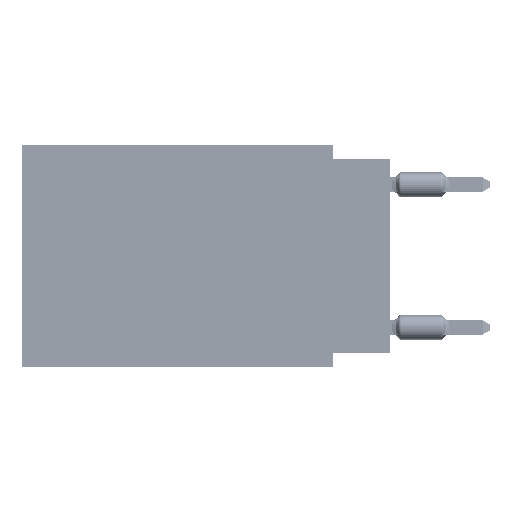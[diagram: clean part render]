
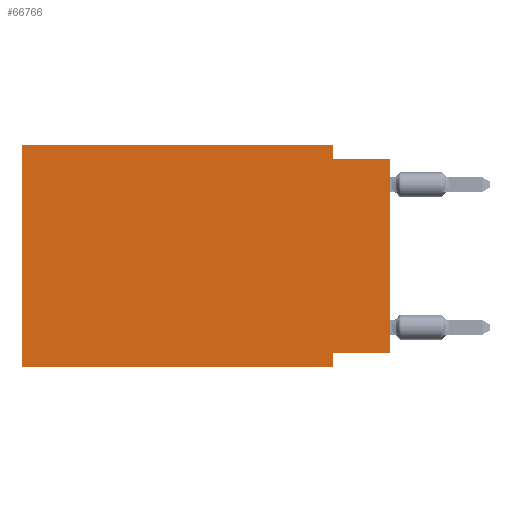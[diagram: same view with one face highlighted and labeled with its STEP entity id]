
A CAD part, left-side view. The second image highlights one B-rep face of the part: STEP entity #66766.
In plain terms, the highlighted planar face has unit normal (-1, 0, 0).
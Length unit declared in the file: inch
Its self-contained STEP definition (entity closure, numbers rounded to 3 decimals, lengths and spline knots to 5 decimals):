
#260 = ORIENTED_EDGE ( 'NONE', *, *, #37451, .T. ) ;
#2139 = DIRECTION ( 'NONE',  ( 0., 0., -1. ) ) ;
#2690 = DIRECTION ( 'NONE',  ( 0., -1., 0. ) ) ;
#2821 = CARTESIAN_POINT ( 'NONE',  ( 0., 0.1, -0.39 ) ) ;
#4115 = VERTEX_POINT ( 'NONE', #2821 ) ;
#4960 = LINE ( 'NONE', #43911, #25141 ) ;
#6924 = ORIENTED_EDGE ( 'NONE', *, *, #10248, .F. ) ;
#7031 = CARTESIAN_POINT ( 'NONE',  ( 0., 0., 0. ) ) ;
#8588 = CARTESIAN_POINT ( 'NONE',  ( 0., 0.1, 0. ) ) ;
#9007 = CARTESIAN_POINT ( 'NONE',  ( 0., 0., -0.025 ) ) ;
#9080 = LINE ( 'NONE', #58769, #21565 ) ;
#9121 = VECTOR ( 'NONE', #60297, 39.37008 ) ;
#9276 = CARTESIAN_POINT ( 'NONE',  ( 0., 0., -0.365 ) ) ;
#9802 = ORIENTED_EDGE ( 'NONE', *, *, #56569, .T. ) ;
#10019 = DIRECTION ( 'NONE',  ( 0., 1., 0. ) ) ;
#10248 = EDGE_CURVE ( 'NONE', #26288, #44771, #20748, .T. ) ;
#11384 = CARTESIAN_POINT ( 'NONE',  ( 0., 0.645, -0.39 ) ) ;
#11724 = CARTESIAN_POINT ( 'NONE',  ( 0., 0.1, 0. ) ) ;
#11728 = CARTESIAN_POINT ( 'NONE',  ( 0., 0.645, -0.39 ) ) ;
#11824 = EDGE_CURVE ( 'NONE', #50966, #15535, #4960, .T. ) ;
#15233 = ORIENTED_EDGE ( 'NONE', *, *, #40867, .F. ) ;
#15535 = VERTEX_POINT ( 'NONE', #11724 ) ;
#15946 = CARTESIAN_POINT ( 'NONE',  ( 0., 0.645, 0. ) ) ;
#15958 = DIRECTION ( 'NONE',  ( 0., 0., 1. ) ) ;
#18775 = CARTESIAN_POINT ( 'NONE',  ( 0., 0., -0.025 ) ) ;
#20002 = EDGE_CURVE ( 'NONE', #15535, #49779, #34676, .T. ) ;
#20748 = LINE ( 'NONE', #42547, #29524 ) ;
#20987 = LINE ( 'NONE', #59203, #32807 ) ;
#21317 = DIRECTION ( 'NONE',  ( 0., 0., -1. ) ) ;
#21565 = VECTOR ( 'NONE', #53057, 39.37008 ) ;
#22765 = LINE ( 'NONE', #7031, #9121 ) ;
#23816 = ORIENTED_EDGE ( 'NONE', *, *, #70513, .F. ) ;
#24324 = VECTOR ( 'NONE', #2139, 39.37008 ) ;
#25141 = VECTOR ( 'NONE', #42475, 39.37008 ) ;
#26288 = VERTEX_POINT ( 'NONE', #9276 ) ;
#28100 = FACE_OUTER_BOUND ( 'NONE', #34383, .T. ) ;
#29524 = VECTOR ( 'NONE', #10019, 39.37008 ) ;
#32807 = VECTOR ( 'NONE', #15958, 39.37008 ) ;
#34383 = EDGE_LOOP ( 'NONE', ( #260, #15233, #36076, #56979, #23816, #9802, #59638, #6924 ) ) ;
#34676 = LINE ( 'NONE', #8588, #24324 ) ;
#36076 = ORIENTED_EDGE ( 'NONE', *, *, #20002, .F. ) ;
#37451 = EDGE_CURVE ( 'NONE', #26288, #57579, #22765, .T. ) ;
#40867 = EDGE_CURVE ( 'NONE', #49779, #57579, #50947, .T. ) ;
#42475 = DIRECTION ( 'NONE',  ( 0., -1., 0. ) ) ;
#42547 = CARTESIAN_POINT ( 'NONE',  ( 0., 0., -0.365 ) ) ;
#43911 = CARTESIAN_POINT ( 'NONE',  ( 0., 0.645, 0. ) ) ;
#44771 = VERTEX_POINT ( 'NONE', #50774 ) ;
#44972 = LINE ( 'NONE', #11728, #56500 ) ;
#45329 = EDGE_CURVE ( 'NONE', #44771, #4115, #9080, .T. ) ;
#46157 = AXIS2_PLACEMENT_3D ( 'NONE', #15946, #70275, #21317 ) ;
#47991 = VERTEX_POINT ( 'NONE', #11384 ) ;
#48225 = VECTOR ( 'NONE', #2690, 39.37008 ) ;
#49586 = CARTESIAN_POINT ( 'NONE',  ( 0., 0.1, -0.025 ) ) ;
#49779 = VERTEX_POINT ( 'NONE', #49586 ) ;
#50774 = CARTESIAN_POINT ( 'NONE',  ( 0., 0.1, -0.365 ) ) ;
#50947 = LINE ( 'NONE', #18775, #48225 ) ;
#50966 = VERTEX_POINT ( 'NONE', #62731 ) ;
#53057 = DIRECTION ( 'NONE',  ( 0., 0., -1. ) ) ;
#56500 = VECTOR ( 'NONE', #61054, 39.37008 ) ;
#56569 = EDGE_CURVE ( 'NONE', #47991, #4115, #44972, .T. ) ;
#56979 = ORIENTED_EDGE ( 'NONE', *, *, #11824, .F. ) ;
#57579 = VERTEX_POINT ( 'NONE', #9007 ) ;
#58769 = CARTESIAN_POINT ( 'NONE',  ( 0., 0.1, -0.39 ) ) ;
#59203 = CARTESIAN_POINT ( 'NONE',  ( 0., 0.645, 0. ) ) ;
#59638 = ORIENTED_EDGE ( 'NONE', *, *, #45329, .F. ) ;
#60297 = DIRECTION ( 'NONE',  ( 0., 0., 1. ) ) ;
#60606 = PLANE ( 'NONE',  #46157 ) ;
#61054 = DIRECTION ( 'NONE',  ( 0., -1., 0. ) ) ;
#62731 = CARTESIAN_POINT ( 'NONE',  ( 0., 0.645, 0. ) ) ;
#66766 = ADVANCED_FACE ( 'NONE', ( #28100 ), #60606, .F. ) ;
#70275 = DIRECTION ( 'NONE',  ( 1., 0., 0. ) ) ;
#70513 = EDGE_CURVE ( 'NONE', #47991, #50966, #20987, .T. ) ;
